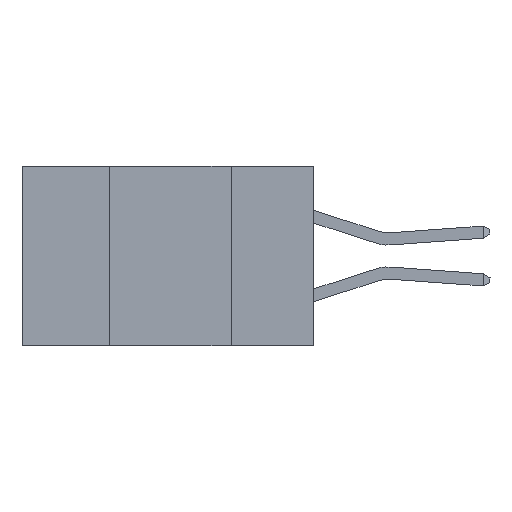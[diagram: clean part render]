
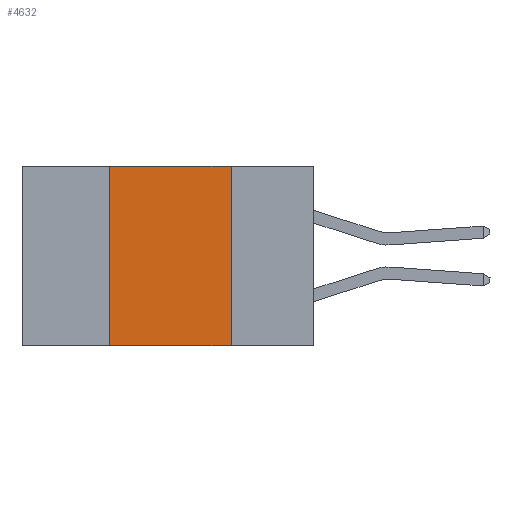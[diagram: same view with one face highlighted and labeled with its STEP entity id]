
A CAD part, left-side view. The second image highlights one B-rep face of the part: STEP entity #4632.
In plain terms, the highlighted planar face has unit normal (-1, 0, 0).
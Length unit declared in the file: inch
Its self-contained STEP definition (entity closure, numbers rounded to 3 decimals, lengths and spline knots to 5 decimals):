
#198 = LINE ( 'NONE', #12199, #10270 ) ;
#370 = EDGE_CURVE ( 'NONE', #2888, #1361, #6974, .T. ) ;
#1026 = EDGE_CURVE ( 'NONE', #11869, #11523, #4861, .T. ) ;
#1283 = EDGE_LOOP ( 'NONE', ( #8148, #1801, #7809, #2097 ) ) ;
#1293 = LINE ( 'NONE', #5862, #9108 ) ;
#1361 = VERTEX_POINT ( 'NONE', #4118 ) ;
#1801 = ORIENTED_EDGE ( 'NONE', *, *, #6049, .F. ) ;
#2097 = ORIENTED_EDGE ( 'NONE', *, *, #3063, .T. ) ;
#2164 = DIRECTION ( 'NONE',  ( 0., -1., 0. ) ) ;
#2888 = VERTEX_POINT ( 'NONE', #7522 ) ;
#3063 = EDGE_CURVE ( 'NONE', #11869, #1361, #1293, .T. ) ;
#3429 = VECTOR ( 'NONE', #11452, 39.37008 ) ;
#3575 = VECTOR ( 'NONE', #4738, 39.37008 ) ;
#3687 = PLANE ( 'NONE',  #8067 ) ;
#4118 = CARTESIAN_POINT ( 'NONE',  ( 0., 0.17, -0.37 ) ) ;
#4632 = ADVANCED_FACE ( 'NONE', ( #8914 ), #3687, .F. ) ;
#4721 = DIRECTION ( 'NONE',  ( 1., 0., 0. ) ) ;
#4738 = DIRECTION ( 'NONE',  ( 0., 0., 1. ) ) ;
#4861 = LINE ( 'NONE', #5666, #3575 ) ;
#5666 = CARTESIAN_POINT ( 'NONE',  ( 0., 0.42, 0. ) ) ;
#5862 = CARTESIAN_POINT ( 'NONE',  ( 0., 0.6, -0.37 ) ) ;
#6049 = EDGE_CURVE ( 'NONE', #11523, #2888, #198, .T. ) ;
#6750 = DIRECTION ( 'NONE',  ( 0., -1., 0. ) ) ;
#6883 = CARTESIAN_POINT ( 'NONE',  ( 0., 0.42, -0.37 ) ) ;
#6974 = LINE ( 'NONE', #11090, #3429 ) ;
#7270 = CARTESIAN_POINT ( 'NONE',  ( 0., 0.42, 0. ) ) ;
#7522 = CARTESIAN_POINT ( 'NONE',  ( 0., 0.17, 0. ) ) ;
#7809 = ORIENTED_EDGE ( 'NONE', *, *, #1026, .F. ) ;
#8067 = AXIS2_PLACEMENT_3D ( 'NONE', #10372, #4721, #11248 ) ;
#8148 = ORIENTED_EDGE ( 'NONE', *, *, #370, .F. ) ;
#8914 = FACE_OUTER_BOUND ( 'NONE', #1283, .T. ) ;
#9108 = VECTOR ( 'NONE', #2164, 39.37008 ) ;
#10270 = VECTOR ( 'NONE', #6750, 39.37008 ) ;
#10372 = CARTESIAN_POINT ( 'NONE',  ( 0., 0.6, 0. ) ) ;
#11090 = CARTESIAN_POINT ( 'NONE',  ( 0., 0.17, 0. ) ) ;
#11248 = DIRECTION ( 'NONE',  ( 0., 0., -1. ) ) ;
#11452 = DIRECTION ( 'NONE',  ( 0., 0., -1. ) ) ;
#11523 = VERTEX_POINT ( 'NONE', #7270 ) ;
#11869 = VERTEX_POINT ( 'NONE', #6883 ) ;
#12199 = CARTESIAN_POINT ( 'NONE',  ( 0., 0.6, 0. ) ) ;
